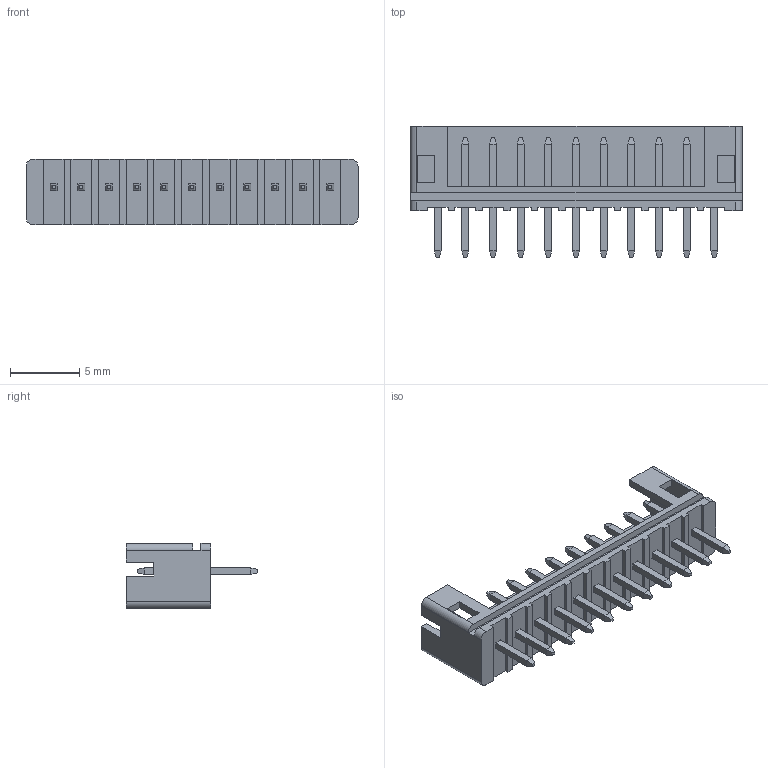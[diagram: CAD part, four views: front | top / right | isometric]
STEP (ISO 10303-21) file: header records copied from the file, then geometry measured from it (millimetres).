
FILE_DESCRIPTION (( 'STEP AP203' ), '1' );
FILE_NAME ('140-511-415-101.STEP', '2020-09-25T11:18:01', ( '' ), ( '' ), 'SwSTEP 2.0', 'SolidWorks 2020', '' );
FILE_SCHEMA (( 'CONFIG_CONTROL_DESIGN' ));
Length unit declared in the file: millimetre
Products named in the file (3): 140-511-415-101; V LI Housing_511; V LI Contact_Str
Assembly tree (12 placements, depth 2):
  140-511-415-101
    V LI Housing_511
    V LI Contact_Str  x11
Bounding box: 24 x 9.5 x 4.7 mm (x, y, z)
Volume: 251.2 mm3; surface area: 918.1 mm2
Topology: 12 solids, 12 shells, 282 faces, 688 edges, 428 vertices
Faces by surface type: plane 276, cylinder 6
Entity records: 5225 total; most frequent: CARTESIAN_POINT 833, ORIENTED_EDGE 816, DIRECTION 734, EDGE_CURVE 408, LINE 396, VECTOR 396, VERTEX_POINT 268, AXIS2_PLACEMENT_3D 169
